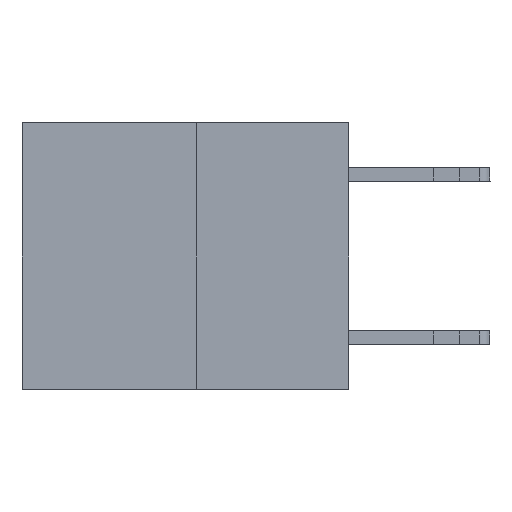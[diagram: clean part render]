
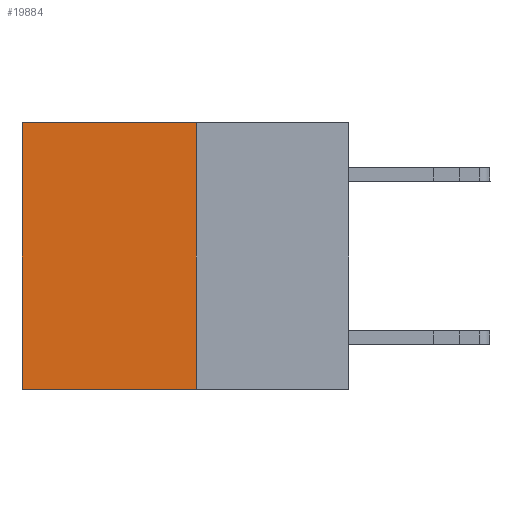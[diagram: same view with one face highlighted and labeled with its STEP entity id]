
A CAD part, left-side view. The second image highlights one B-rep face of the part: STEP entity #19884.
In plain terms, the highlighted planar face has unit normal (-1, 0, 0).
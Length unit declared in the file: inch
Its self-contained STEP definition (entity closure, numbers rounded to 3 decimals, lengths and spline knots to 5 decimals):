
#234 = ORIENTED_EDGE ( 'NONE', *, *, #12730, .F. ) ;
#261 = LINE ( 'NONE', #17057, #23066 ) ;
#730 = DIRECTION ( 'NONE',  ( 0., 0., -1. ) ) ;
#839 = VECTOR ( 'NONE', #11274, 39.37008 ) ;
#2851 = CARTESIAN_POINT ( 'NONE',  ( 0.3165, 0.28, -0.49 ) ) ;
#2889 = VERTEX_POINT ( 'NONE', #11733 ) ;
#2957 = CARTESIAN_POINT ( 'NONE',  ( 0.3165, 0.28, -0.49 ) ) ;
#2978 = VECTOR ( 'NONE', #8562, 39.37008 ) ;
#4486 = CARTESIAN_POINT ( 'NONE',  ( 0.3165, 0.28, -0.49 ) ) ;
#4600 = DIRECTION ( 'NONE',  ( 0., 1., 0. ) ) ;
#7046 = EDGE_LOOP ( 'NONE', ( #23974, #20988, #234, #23693 ) ) ;
#7082 = CARTESIAN_POINT ( 'NONE',  ( 0.3165, 0.6, -0.49 ) ) ;
#8562 = DIRECTION ( 'NONE',  ( 0., 0., -1. ) ) ;
#8998 = LINE ( 'NONE', #7082, #839 ) ;
#9149 = VERTEX_POINT ( 'NONE', #10646 ) ;
#9501 = CARTESIAN_POINT ( 'NONE',  ( 0.3165, 0.28, -0.49 ) ) ;
#9559 = VECTOR ( 'NONE', #25873, 39.37008 ) ;
#10415 = AXIS2_PLACEMENT_3D ( 'NONE', #2851, #17394, #730 ) ;
#10646 = CARTESIAN_POINT ( 'NONE',  ( 0.3165, 0.28, 0. ) ) ;
#11265 = EDGE_CURVE ( 'NONE', #17037, #23749, #21307, .T. ) ;
#11274 = DIRECTION ( 'NONE',  ( 0., 0., -1. ) ) ;
#11733 = CARTESIAN_POINT ( 'NONE',  ( 0.3165, 0.6, 0. ) ) ;
#12730 = EDGE_CURVE ( 'NONE', #9149, #17037, #18908, .T. ) ;
#13706 = EDGE_CURVE ( 'NONE', #9149, #2889, #261, .T. ) ;
#17037 = VERTEX_POINT ( 'NONE', #9501 ) ;
#17057 = CARTESIAN_POINT ( 'NONE',  ( 0.3165, 0.28, 0. ) ) ;
#17386 = FACE_OUTER_BOUND ( 'NONE', #7046, .T. ) ;
#17394 = DIRECTION ( 'NONE',  ( 1., 0., 0. ) ) ;
#17653 = PLANE ( 'NONE',  #10415 ) ;
#18053 = EDGE_CURVE ( 'NONE', #2889, #23749, #8998, .T. ) ;
#18908 = LINE ( 'NONE', #4486, #2978 ) ;
#19884 = ADVANCED_FACE ( 'NONE', ( #17386 ), #17653, .F. ) ;
#20988 = ORIENTED_EDGE ( 'NONE', *, *, #11265, .F. ) ;
#21307 = LINE ( 'NONE', #2957, #9559 ) ;
#23066 = VECTOR ( 'NONE', #4600, 39.37008 ) ;
#23693 = ORIENTED_EDGE ( 'NONE', *, *, #13706, .T. ) ;
#23749 = VERTEX_POINT ( 'NONE', #23923 ) ;
#23923 = CARTESIAN_POINT ( 'NONE',  ( 0.3165, 0.6, -0.49 ) ) ;
#23974 = ORIENTED_EDGE ( 'NONE', *, *, #18053, .T. ) ;
#25873 = DIRECTION ( 'NONE',  ( 0., 1., 0. ) ) ;
